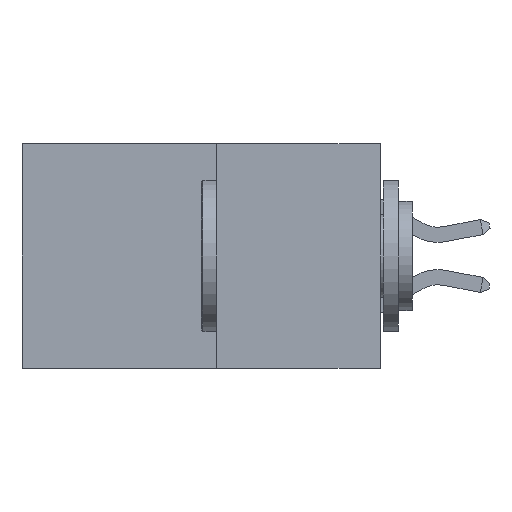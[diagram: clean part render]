
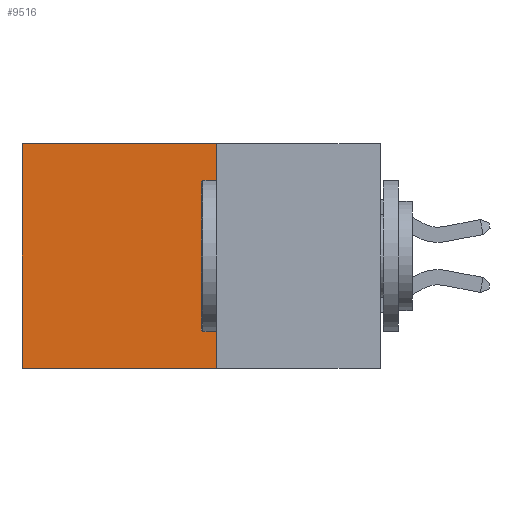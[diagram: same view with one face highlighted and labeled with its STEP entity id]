
A CAD part, left-side view. The second image highlights one B-rep face of the part: STEP entity #9516.
In plain terms, the highlighted planar face has unit normal (-1, 0, 0).
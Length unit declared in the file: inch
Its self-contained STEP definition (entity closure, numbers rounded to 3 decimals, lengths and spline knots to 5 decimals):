
#933 = DIRECTION ( 'NONE',  ( 1., 0., 0. ) ) ;
#1057 = EDGE_LOOP ( 'NONE', ( #9020, #11652, #9320, #11952 ) ) ;
#1553 = EDGE_CURVE ( 'NONE', #12576, #7968, #12105, .T. ) ;
#1797 = EDGE_CURVE ( 'NONE', #9815, #12201, #12684, .T. ) ;
#1857 = VECTOR ( 'NONE', #3822, 39.37008 ) ;
#2122 = CARTESIAN_POINT ( 'NONE',  ( 0.277, 0.27, 0. ) ) ;
#2278 = DIRECTION ( 'NONE',  ( 0., 0., -1. ) ) ;
#2614 = DIRECTION ( 'NONE',  ( 0., 0., -1. ) ) ;
#3199 = EDGE_CURVE ( 'NONE', #9815, #12576, #12034, .T. ) ;
#3780 = CARTESIAN_POINT ( 'NONE',  ( 0.277, 0.59, -0.37 ) ) ;
#3822 = DIRECTION ( 'NONE',  ( 0., 1., 0. ) ) ;
#3924 = VECTOR ( 'NONE', #7247, 39.37008 ) ;
#4534 = AXIS2_PLACEMENT_3D ( 'NONE', #8694, #933, #8732 ) ;
#4557 = CARTESIAN_POINT ( 'NONE',  ( 0.277, 0.27, -0.37 ) ) ;
#5675 = VECTOR ( 'NONE', #2278, 39.37008 ) ;
#6928 = CARTESIAN_POINT ( 'NONE',  ( 0.277, 0.27, 0. ) ) ;
#6991 = CARTESIAN_POINT ( 'NONE',  ( 0.277, 0.59, -0.37 ) ) ;
#7247 = DIRECTION ( 'NONE',  ( 0., 1., 0. ) ) ;
#7362 = CARTESIAN_POINT ( 'NONE',  ( 0.277, 0.27, -0.37 ) ) ;
#7968 = VERTEX_POINT ( 'NONE', #3780 ) ;
#8694 = CARTESIAN_POINT ( 'NONE',  ( 0.277, 0.27, -0.37 ) ) ;
#8732 = DIRECTION ( 'NONE',  ( 0., 0., -1. ) ) ;
#8911 = EDGE_CURVE ( 'NONE', #12201, #7968, #10527, .T. ) ;
#9020 = ORIENTED_EDGE ( 'NONE', *, *, #8911, .T. ) ;
#9320 = ORIENTED_EDGE ( 'NONE', *, *, #3199, .F. ) ;
#9516 = ADVANCED_FACE ( 'NONE', ( #11765 ), #13605, .F. ) ;
#9815 = VERTEX_POINT ( 'NONE', #6928 ) ;
#9822 = CARTESIAN_POINT ( 'NONE',  ( 0.277, 0.59, 0. ) ) ;
#10296 = CARTESIAN_POINT ( 'NONE',  ( 0.277, 0.27, -0.37 ) ) ;
#10527 = LINE ( 'NONE', #6991, #12814 ) ;
#11652 = ORIENTED_EDGE ( 'NONE', *, *, #1553, .F. ) ;
#11765 = FACE_OUTER_BOUND ( 'NONE', #1057, .T. ) ;
#11952 = ORIENTED_EDGE ( 'NONE', *, *, #1797, .T. ) ;
#12034 = LINE ( 'NONE', #4557, #5675 ) ;
#12105 = LINE ( 'NONE', #7362, #3924 ) ;
#12201 = VERTEX_POINT ( 'NONE', #9822 ) ;
#12576 = VERTEX_POINT ( 'NONE', #10296 ) ;
#12684 = LINE ( 'NONE', #2122, #1857 ) ;
#12814 = VECTOR ( 'NONE', #2614, 39.37008 ) ;
#13605 = PLANE ( 'NONE',  #4534 ) ;
